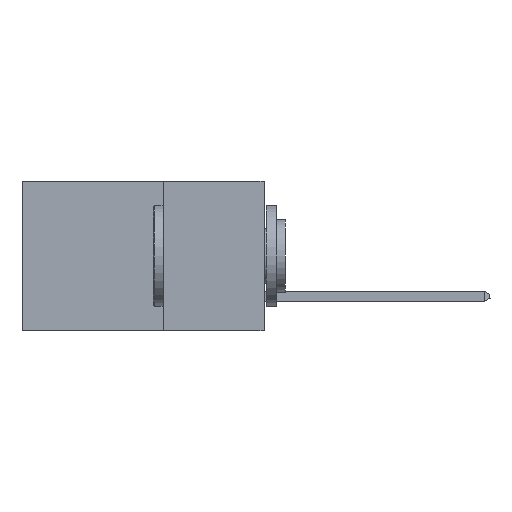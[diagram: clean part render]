
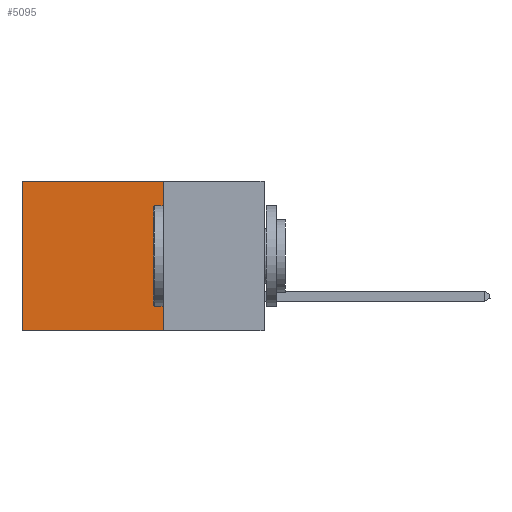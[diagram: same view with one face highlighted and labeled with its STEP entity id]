
A CAD part, left-side view. The second image highlights one B-rep face of the part: STEP entity #5095.
In plain terms, the highlighted planar face has unit normal (-1, 0, 0).
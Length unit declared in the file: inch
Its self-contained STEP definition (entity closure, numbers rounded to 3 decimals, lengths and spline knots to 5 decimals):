
#287 = AXIS2_PLACEMENT_3D ( 'NONE', #8579, #3489, #3561 ) ;
#816 = ORIENTED_EDGE ( 'NONE', *, *, #9170, .T. ) ;
#988 = LINE ( 'NONE', #3710, #3407 ) ;
#1533 = CARTESIAN_POINT ( 'NONE',  ( 0.298, 0.25, -0.37 ) ) ;
#1719 = EDGE_LOOP ( 'NONE', ( #816, #4975, #10423, #2045 ) ) ;
#1962 = LINE ( 'NONE', #5482, #10760 ) ;
#2045 = ORIENTED_EDGE ( 'NONE', *, *, #3395, .T. ) ;
#2214 = VECTOR ( 'NONE', #9754, 39.37008 ) ;
#2942 = CARTESIAN_POINT ( 'NONE',  ( 0.298, 0.6, 0. ) ) ;
#3158 = DIRECTION ( 'NONE',  ( 0., 0., -1. ) ) ;
#3395 = EDGE_CURVE ( 'NONE', #7682, #7870, #3570, .T. ) ;
#3407 = VECTOR ( 'NONE', #7272, 39.37008 ) ;
#3489 = DIRECTION ( 'NONE',  ( 1., 0., 0. ) ) ;
#3561 = DIRECTION ( 'NONE',  ( 0., 0., -1. ) ) ;
#3570 = LINE ( 'NONE', #8785, #2214 ) ;
#3710 = CARTESIAN_POINT ( 'NONE',  ( 0.298, 0.25, 0. ) ) ;
#4059 = CARTESIAN_POINT ( 'NONE',  ( 0.298, 0.25, 0. ) ) ;
#4820 = EDGE_CURVE ( 'NONE', #7682, #7905, #988, .T. ) ;
#4975 = ORIENTED_EDGE ( 'NONE', *, *, #10227, .F. ) ;
#5095 = ADVANCED_FACE ( 'NONE', ( #6441 ), #9434, .F. ) ;
#5482 = CARTESIAN_POINT ( 'NONE',  ( 0.298, 0.25, -0.37 ) ) ;
#6053 = VERTEX_POINT ( 'NONE', #9169 ) ;
#6441 = FACE_OUTER_BOUND ( 'NONE', #1719, .T. ) ;
#6906 = VECTOR ( 'NONE', #3158, 39.37008 ) ;
#7272 = DIRECTION ( 'NONE',  ( 0., 0., -1. ) ) ;
#7682 = VERTEX_POINT ( 'NONE', #4059 ) ;
#7870 = VERTEX_POINT ( 'NONE', #2942 ) ;
#7905 = VERTEX_POINT ( 'NONE', #1533 ) ;
#8579 = CARTESIAN_POINT ( 'NONE',  ( 0.298, 0.25, 0. ) ) ;
#8785 = CARTESIAN_POINT ( 'NONE',  ( 0.298, 0.25, 0. ) ) ;
#9169 = CARTESIAN_POINT ( 'NONE',  ( 0.298, 0.6, -0.37 ) ) ;
#9170 = EDGE_CURVE ( 'NONE', #7870, #6053, #9181, .T. ) ;
#9181 = LINE ( 'NONE', #9201, #6906 ) ;
#9201 = CARTESIAN_POINT ( 'NONE',  ( 0.298, 0.6, 0. ) ) ;
#9434 = PLANE ( 'NONE',  #287 ) ;
#9709 = DIRECTION ( 'NONE',  ( 0., 1., 0. ) ) ;
#9754 = DIRECTION ( 'NONE',  ( 0., 1., 0. ) ) ;
#10227 = EDGE_CURVE ( 'NONE', #7905, #6053, #1962, .T. ) ;
#10423 = ORIENTED_EDGE ( 'NONE', *, *, #4820, .F. ) ;
#10760 = VECTOR ( 'NONE', #9709, 39.37008 ) ;
